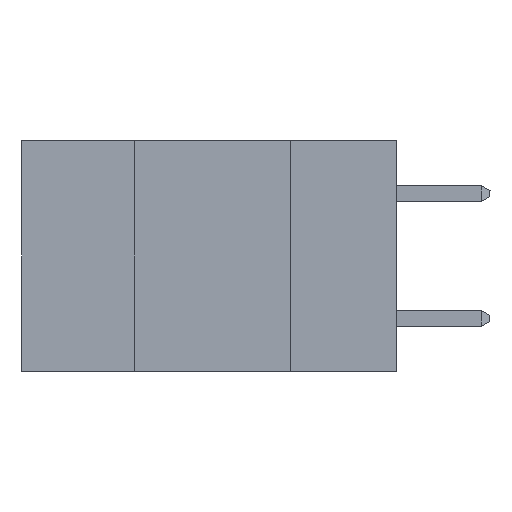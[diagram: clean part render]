
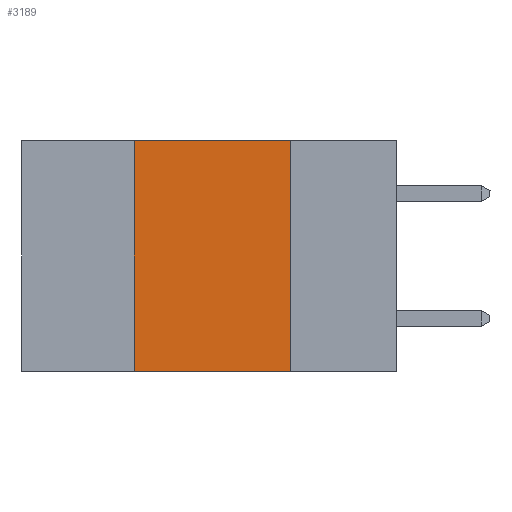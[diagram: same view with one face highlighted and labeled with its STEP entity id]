
A CAD part, left-side view. The second image highlights one B-rep face of the part: STEP entity #3189.
In plain terms, the highlighted planar face has unit normal (-1, 0, 0).
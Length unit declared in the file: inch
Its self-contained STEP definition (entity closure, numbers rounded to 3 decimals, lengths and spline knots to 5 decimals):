
#128 = EDGE_LOOP ( 'NONE', ( #10362, #757, #2055, #6122 ) ) ;
#425 = CARTESIAN_POINT ( 'NONE',  ( 0., 0.6, -0.37 ) ) ;
#499 = EDGE_CURVE ( 'NONE', #1852, #4352, #9292, .T. ) ;
#623 = CARTESIAN_POINT ( 'NONE',  ( 0., 0.42, -0.37 ) ) ;
#757 = ORIENTED_EDGE ( 'NONE', *, *, #4017, .F. ) ;
#1740 = PLANE ( 'NONE',  #8889 ) ;
#1852 = VERTEX_POINT ( 'NONE', #623 ) ;
#1861 = LINE ( 'NONE', #2000, #5882 ) ;
#1923 = VERTEX_POINT ( 'NONE', #9883 ) ;
#1948 = DIRECTION ( 'NONE',  ( 0., 0., -1. ) ) ;
#2000 = CARTESIAN_POINT ( 'NONE',  ( 0., 0.42, 0. ) ) ;
#2055 = ORIENTED_EDGE ( 'NONE', *, *, #8878, .F. ) ;
#2344 = LINE ( 'NONE', #6968, #2642 ) ;
#2531 = FACE_OUTER_BOUND ( 'NONE', #128, .T. ) ;
#2642 = VECTOR ( 'NONE', #1948, 39.37008 ) ;
#3189 = ADVANCED_FACE ( 'NONE', ( #2531 ), #1740, .F. ) ;
#3199 = DIRECTION ( 'NONE',  ( 1., 0., 0. ) ) ;
#3213 = DIRECTION ( 'NONE',  ( 0., 0., -1. ) ) ;
#3989 = CARTESIAN_POINT ( 'NONE',  ( 0., 0.6, 0. ) ) ;
#4017 = EDGE_CURVE ( 'NONE', #1923, #7215, #5664, .T. ) ;
#4352 = VERTEX_POINT ( 'NONE', #9654 ) ;
#5664 = LINE ( 'NONE', #3989, #9553 ) ;
#5882 = VECTOR ( 'NONE', #7801, 39.37008 ) ;
#6030 = DIRECTION ( 'NONE',  ( 0., -1., 0. ) ) ;
#6122 = ORIENTED_EDGE ( 'NONE', *, *, #499, .T. ) ;
#6447 = CARTESIAN_POINT ( 'NONE',  ( 0., 0.6, 0. ) ) ;
#6968 = CARTESIAN_POINT ( 'NONE',  ( 0., 0.17, 0. ) ) ;
#7213 = VECTOR ( 'NONE', #6030, 39.37008 ) ;
#7215 = VERTEX_POINT ( 'NONE', #9208 ) ;
#7712 = DIRECTION ( 'NONE',  ( 0., -1., 0. ) ) ;
#7801 = DIRECTION ( 'NONE',  ( 0., 0., 1. ) ) ;
#8878 = EDGE_CURVE ( 'NONE', #1852, #1923, #1861, .T. ) ;
#8889 = AXIS2_PLACEMENT_3D ( 'NONE', #6447, #3199, #3213 ) ;
#9208 = CARTESIAN_POINT ( 'NONE',  ( 0., 0.17, 0. ) ) ;
#9292 = LINE ( 'NONE', #425, #7213 ) ;
#9549 = EDGE_CURVE ( 'NONE', #7215, #4352, #2344, .T. ) ;
#9553 = VECTOR ( 'NONE', #7712, 39.37008 ) ;
#9654 = CARTESIAN_POINT ( 'NONE',  ( 0., 0.17, -0.37 ) ) ;
#9883 = CARTESIAN_POINT ( 'NONE',  ( 0., 0.42, 0. ) ) ;
#10362 = ORIENTED_EDGE ( 'NONE', *, *, #9549, .F. ) ;
